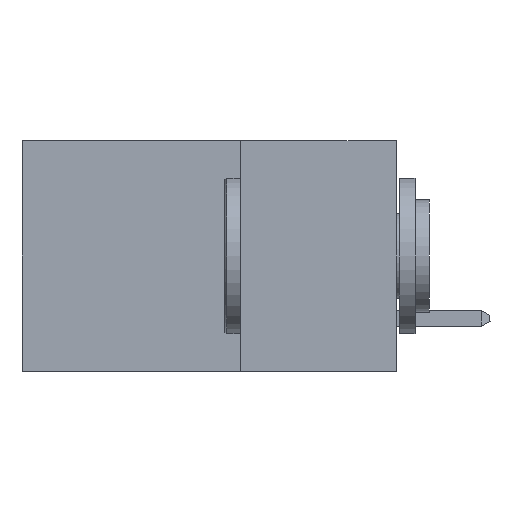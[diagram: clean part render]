
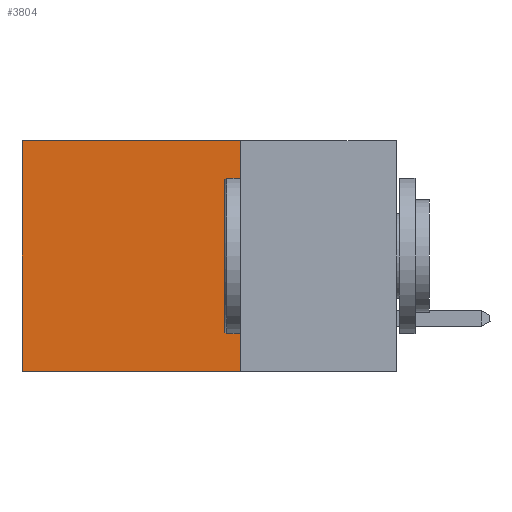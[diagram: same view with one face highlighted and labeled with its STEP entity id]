
A CAD part, left-side view. The second image highlights one B-rep face of the part: STEP entity #3804.
In plain terms, the highlighted planar face has unit normal (-1, 0, 0).
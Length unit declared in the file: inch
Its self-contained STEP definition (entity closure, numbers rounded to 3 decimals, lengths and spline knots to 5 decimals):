
#153 = VECTOR ( 'NONE', #30043, 39.37008 ) ;
#1001 = FACE_OUTER_BOUND ( 'NONE', #32367, .T. ) ;
#1931 = CARTESIAN_POINT ( 'NONE',  ( 0.298, 0.25, -0.37 ) ) ;
#3305 = CARTESIAN_POINT ( 'NONE',  ( 0.298, 0.6, 0. ) ) ;
#3804 = ADVANCED_FACE ( 'NONE', ( #1001 ), #17352, .F. ) ;
#4384 = DIRECTION ( 'NONE',  ( 0., 1., 0. ) ) ;
#4668 = EDGE_CURVE ( 'NONE', #22251, #12958, #19581, .T. ) ;
#5405 = EDGE_CURVE ( 'NONE', #15163, #12221, #15461, .T. ) ;
#6030 = LINE ( 'NONE', #24759, #24763 ) ;
#8453 = LINE ( 'NONE', #1931, #18529 ) ;
#10881 = EDGE_CURVE ( 'NONE', #12221, #12958, #8453, .T. ) ;
#11767 = CARTESIAN_POINT ( 'NONE',  ( 0.298, 0.6, -0.37 ) ) ;
#12221 = VERTEX_POINT ( 'NONE', #16873 ) ;
#12936 = DIRECTION ( 'NONE',  ( 0., 0., -1. ) ) ;
#12958 = VERTEX_POINT ( 'NONE', #11767 ) ;
#15163 = VERTEX_POINT ( 'NONE', #17766 ) ;
#15461 = LINE ( 'NONE', #30524, #22256 ) ;
#16873 = CARTESIAN_POINT ( 'NONE',  ( 0.298, 0.25, -0.37 ) ) ;
#16930 = CARTESIAN_POINT ( 'NONE',  ( 0.298, 0.25, 0. ) ) ;
#17352 = PLANE ( 'NONE',  #19772 ) ;
#17403 = ORIENTED_EDGE ( 'NONE', *, *, #5405, .F. ) ;
#17766 = CARTESIAN_POINT ( 'NONE',  ( 0.298, 0.25, 0. ) ) ;
#17838 = ORIENTED_EDGE ( 'NONE', *, *, #4668, .T. ) ;
#18480 = ORIENTED_EDGE ( 'NONE', *, *, #10881, .F. ) ;
#18529 = VECTOR ( 'NONE', #4384, 39.37008 ) ;
#19407 = ORIENTED_EDGE ( 'NONE', *, *, #27885, .T. ) ;
#19581 = LINE ( 'NONE', #21229, #153 ) ;
#19590 = DIRECTION ( 'NONE',  ( 0., 0., -1. ) ) ;
#19772 = AXIS2_PLACEMENT_3D ( 'NONE', #16930, #29543, #19590 ) ;
#19840 = DIRECTION ( 'NONE',  ( 0., 1., 0. ) ) ;
#21229 = CARTESIAN_POINT ( 'NONE',  ( 0.298, 0.6, 0. ) ) ;
#22251 = VERTEX_POINT ( 'NONE', #3305 ) ;
#22256 = VECTOR ( 'NONE', #12936, 39.37008 ) ;
#24759 = CARTESIAN_POINT ( 'NONE',  ( 0.298, 0.25, 0. ) ) ;
#24763 = VECTOR ( 'NONE', #19840, 39.37008 ) ;
#27885 = EDGE_CURVE ( 'NONE', #15163, #22251, #6030, .T. ) ;
#29543 = DIRECTION ( 'NONE',  ( 1., 0., 0. ) ) ;
#30043 = DIRECTION ( 'NONE',  ( 0., 0., -1. ) ) ;
#30524 = CARTESIAN_POINT ( 'NONE',  ( 0.298, 0.25, 0. ) ) ;
#32367 = EDGE_LOOP ( 'NONE', ( #17838, #18480, #17403, #19407 ) ) ;
